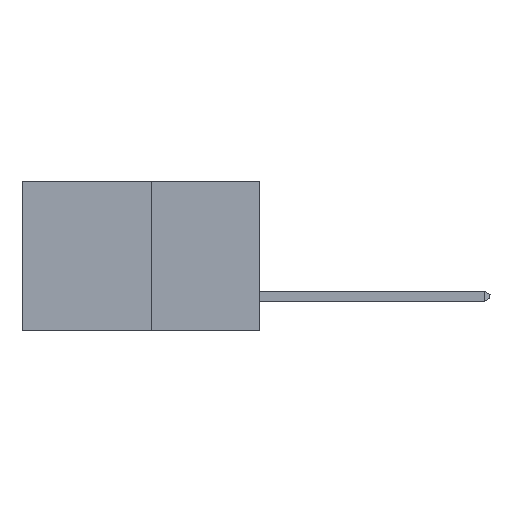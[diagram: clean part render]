
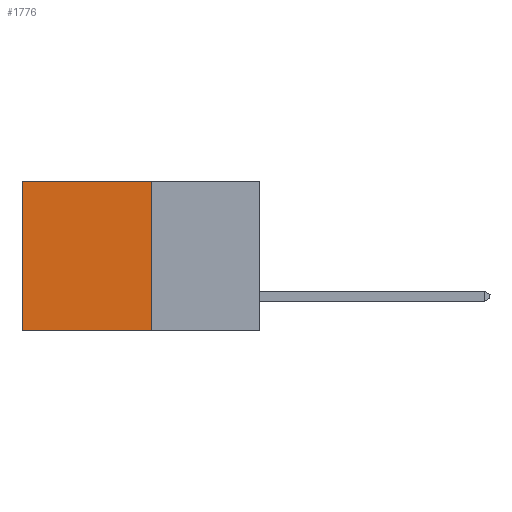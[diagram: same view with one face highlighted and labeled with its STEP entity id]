
A CAD part, left-side view. The second image highlights one B-rep face of the part: STEP entity #1776.
In plain terms, the highlighted planar face has unit normal (-1, 0, 0).
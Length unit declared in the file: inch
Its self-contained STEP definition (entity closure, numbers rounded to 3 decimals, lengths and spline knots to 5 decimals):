
#3 = CARTESIAN_POINT ( 'NONE',  ( 0.277, 0.27, 0. ) ) ;
#120 = EDGE_CURVE ( 'NONE', #1124, #10985, #7424, .T. ) ;
#153 = DIRECTION ( 'NONE',  ( 0., 0., -1. ) ) ;
#373 = EDGE_CURVE ( 'NONE', #3703, #3355, #6007, .T. ) ;
#966 = CARTESIAN_POINT ( 'NONE',  ( 0.277, 0.27, -0.37 ) ) ;
#982 = CARTESIAN_POINT ( 'NONE',  ( 0.277, 0.59, -0.37 ) ) ;
#1116 = DIRECTION ( 'NONE',  ( 0., 0., -1. ) ) ;
#1124 = VERTEX_POINT ( 'NONE', #6931 ) ;
#1368 = DIRECTION ( 'NONE',  ( 0., 1., 0. ) ) ;
#1776 = ADVANCED_FACE ( 'NONE', ( #10683 ), #8443, .F. ) ;
#2405 = EDGE_CURVE ( 'NONE', #1124, #3703, #9777, .T. ) ;
#3097 = AXIS2_PLACEMENT_3D ( 'NONE', #8139, #10433, #153 ) ;
#3355 = VERTEX_POINT ( 'NONE', #982 ) ;
#3703 = VERTEX_POINT ( 'NONE', #7142 ) ;
#3892 = ORIENTED_EDGE ( 'NONE', *, *, #120, .F. ) ;
#5194 = VECTOR ( 'NONE', #1116, 39.37008 ) ;
#6007 = LINE ( 'NONE', #9180, #9700 ) ;
#6931 = CARTESIAN_POINT ( 'NONE',  ( 0.277, 0.27, 0. ) ) ;
#7043 = ORIENTED_EDGE ( 'NONE', *, *, #2405, .T. ) ;
#7142 = CARTESIAN_POINT ( 'NONE',  ( 0.277, 0.59, 0. ) ) ;
#7414 = CARTESIAN_POINT ( 'NONE',  ( 0.277, 0.27, -0.37 ) ) ;
#7424 = LINE ( 'NONE', #966, #5194 ) ;
#7436 = ORIENTED_EDGE ( 'NONE', *, *, #7808, .F. ) ;
#7808 = EDGE_CURVE ( 'NONE', #10985, #3355, #10604, .T. ) ;
#8139 = CARTESIAN_POINT ( 'NONE',  ( 0.277, 0.27, -0.37 ) ) ;
#8274 = EDGE_LOOP ( 'NONE', ( #8399, #7436, #3892, #7043 ) ) ;
#8399 = ORIENTED_EDGE ( 'NONE', *, *, #373, .T. ) ;
#8443 = PLANE ( 'NONE',  #3097 ) ;
#8672 = VECTOR ( 'NONE', #9948, 39.37008 ) ;
#9180 = CARTESIAN_POINT ( 'NONE',  ( 0.277, 0.59, -0.37 ) ) ;
#9225 = CARTESIAN_POINT ( 'NONE',  ( 0.277, 0.27, -0.37 ) ) ;
#9613 = DIRECTION ( 'NONE',  ( 0., 0., -1. ) ) ;
#9700 = VECTOR ( 'NONE', #9613, 39.37008 ) ;
#9777 = LINE ( 'NONE', #3, #10010 ) ;
#9948 = DIRECTION ( 'NONE',  ( 0., 1., 0. ) ) ;
#10010 = VECTOR ( 'NONE', #1368, 39.37008 ) ;
#10433 = DIRECTION ( 'NONE',  ( 1., 0., 0. ) ) ;
#10604 = LINE ( 'NONE', #9225, #8672 ) ;
#10683 = FACE_OUTER_BOUND ( 'NONE', #8274, .T. ) ;
#10985 = VERTEX_POINT ( 'NONE', #7414 ) ;
